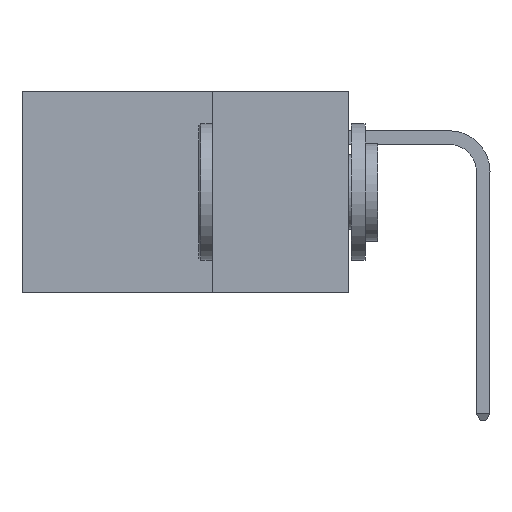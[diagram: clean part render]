
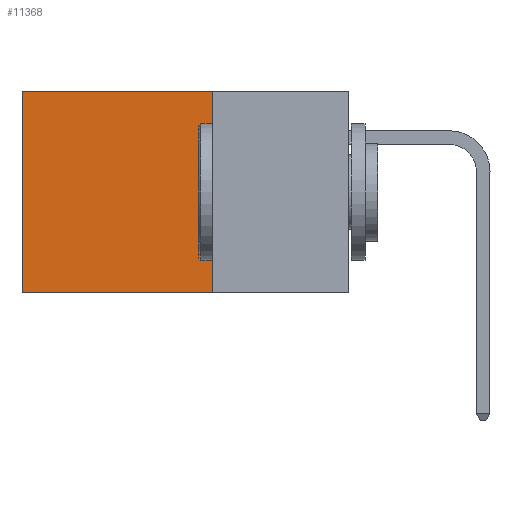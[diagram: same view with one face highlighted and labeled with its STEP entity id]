
A CAD part, left-side view. The second image highlights one B-rep face of the part: STEP entity #11368.
In plain terms, the highlighted planar face has unit normal (-1, 0, 0).
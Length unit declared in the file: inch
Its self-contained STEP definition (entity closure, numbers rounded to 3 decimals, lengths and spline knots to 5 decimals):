
#560 = DIRECTION ( 'NONE',  ( 0., 1., 0. ) ) ;
#4097 = CARTESIAN_POINT ( 'NONE',  ( 0.2875, 0.25, 0. ) ) ;
#5401 = LINE ( 'NONE', #15002, #12171 ) ;
#5573 = ORIENTED_EDGE ( 'NONE', *, *, #19079, .F. ) ;
#6686 = EDGE_CURVE ( 'NONE', #26617, #16724, #23914, .T. ) ;
#7172 = DIRECTION ( 'NONE',  ( 1., 0., 0. ) ) ;
#9653 = CARTESIAN_POINT ( 'NONE',  ( 0.2875, 0.6, -0.37 ) ) ;
#9940 = CARTESIAN_POINT ( 'NONE',  ( 0.2875, 0.25, 0. ) ) ;
#11252 = VECTOR ( 'NONE', #16734, 39.37008 ) ;
#11368 = ADVANCED_FACE ( 'NONE', ( #18499 ), #24243, .F. ) ;
#11569 = EDGE_CURVE ( 'NONE', #18397, #18074, #33775, .T. ) ;
#12171 = VECTOR ( 'NONE', #560, 39.37008 ) ;
#14221 = CARTESIAN_POINT ( 'NONE',  ( 0.2875, 0.25, -0.37 ) ) ;
#14610 = VECTOR ( 'NONE', #15614, 39.37008 ) ;
#15002 = CARTESIAN_POINT ( 'NONE',  ( 0.2875, 0.25, 0. ) ) ;
#15614 = DIRECTION ( 'NONE',  ( 0., 0., -1. ) ) ;
#16111 = EDGE_LOOP ( 'NONE', ( #29890, #5573, #21393, #31099 ) ) ;
#16724 = VERTEX_POINT ( 'NONE', #32373 ) ;
#16734 = DIRECTION ( 'NONE',  ( 0., 0., -1. ) ) ;
#17149 = DIRECTION ( 'NONE',  ( 0., 1., 0. ) ) ;
#18074 = VERTEX_POINT ( 'NONE', #9653 ) ;
#18397 = VERTEX_POINT ( 'NONE', #30971 ) ;
#18499 = FACE_OUTER_BOUND ( 'NONE', #16111, .T. ) ;
#19079 = EDGE_CURVE ( 'NONE', #16724, #18074, #34205, .T. ) ;
#19349 = VECTOR ( 'NONE', #17149, 39.37008 ) ;
#21393 = ORIENTED_EDGE ( 'NONE', *, *, #6686, .F. ) ;
#23565 = EDGE_CURVE ( 'NONE', #26617, #18397, #5401, .T. ) ;
#23914 = LINE ( 'NONE', #4097, #14610 ) ;
#24243 = PLANE ( 'NONE',  #28214 ) ;
#26617 = VERTEX_POINT ( 'NONE', #27536 ) ;
#27068 = DIRECTION ( 'NONE',  ( 0., 0., -1. ) ) ;
#27536 = CARTESIAN_POINT ( 'NONE',  ( 0.2875, 0.25, 0. ) ) ;
#28214 = AXIS2_PLACEMENT_3D ( 'NONE', #9940, #7172, #27068 ) ;
#29890 = ORIENTED_EDGE ( 'NONE', *, *, #11569, .T. ) ;
#30783 = CARTESIAN_POINT ( 'NONE',  ( 0.2875, 0.6, 0. ) ) ;
#30971 = CARTESIAN_POINT ( 'NONE',  ( 0.2875, 0.6, 0. ) ) ;
#31099 = ORIENTED_EDGE ( 'NONE', *, *, #23565, .T. ) ;
#32373 = CARTESIAN_POINT ( 'NONE',  ( 0.2875, 0.25, -0.37 ) ) ;
#33775 = LINE ( 'NONE', #30783, #11252 ) ;
#34205 = LINE ( 'NONE', #14221, #19349 ) ;
